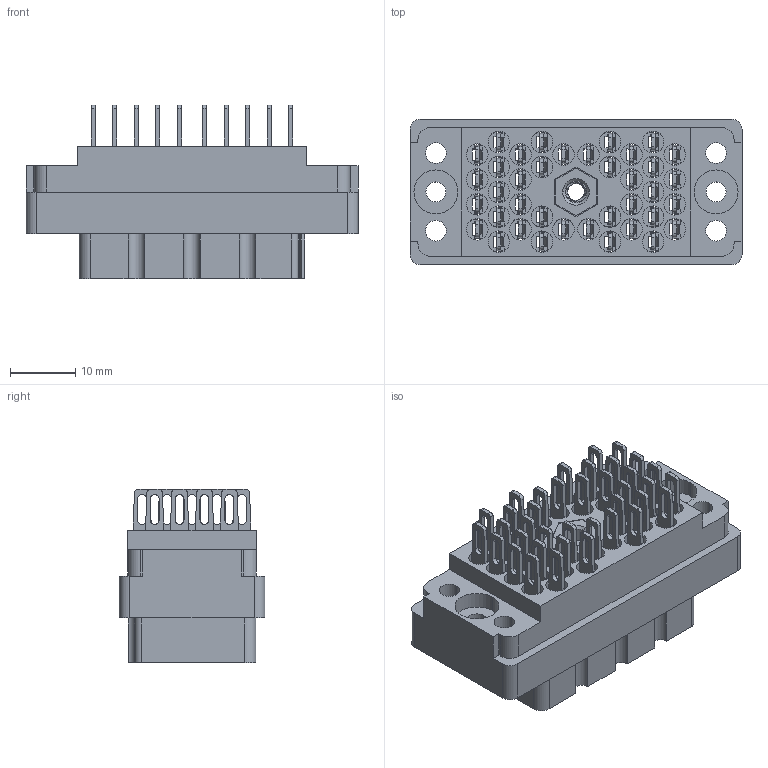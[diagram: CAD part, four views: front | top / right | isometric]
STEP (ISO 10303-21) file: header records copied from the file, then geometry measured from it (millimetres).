
FILE_DESCRIPTION (( 'STEP AP203' ), '1' );
FILE_NAME ('516-038-500-406.STEP', '2020-03-05T12:05:47', ( '' ), ( '' ), 'SwSTEP 2.0', 'SolidWorks 2016', '' );
FILE_SCHEMA (( 'CONFIG_CONTROL_DESIGN' ));
Length unit declared in the file: inch
Products named in the file (4): 516-292-001_500 Contact; 516 Part Receptacle_038; 516-038-500-406; 516-252-035-100_516-252-035-100
Assembly tree (40 placements, depth 2):
  516-038-500-406
    516 Part Receptacle_038
    516-292-001_500 Contact  x38
    516-252-035-100_516-252-035-100
Bounding box: 50.8 x 22.25 x 26.49 mm (x, y, z)
Volume: 12135.2 mm3; surface area: 21752.7 mm2
Topology: 40 solids, 40 shells, 3858 faces, 11194 edges, 7434 vertices
Faces by surface type: plane 2282, cylinder 1330, bspline 234, cone 12
Entity records: 38938 total; most frequent: CARTESIAN_POINT 8906, ORIENTED_EDGE 6108, DIRECTION 5919, EDGE_CURVE 3054, VECTOR 2175, LINE 2175, VERTEX_POINT 2032, AXIS2_PLACEMENT_3D 1872
